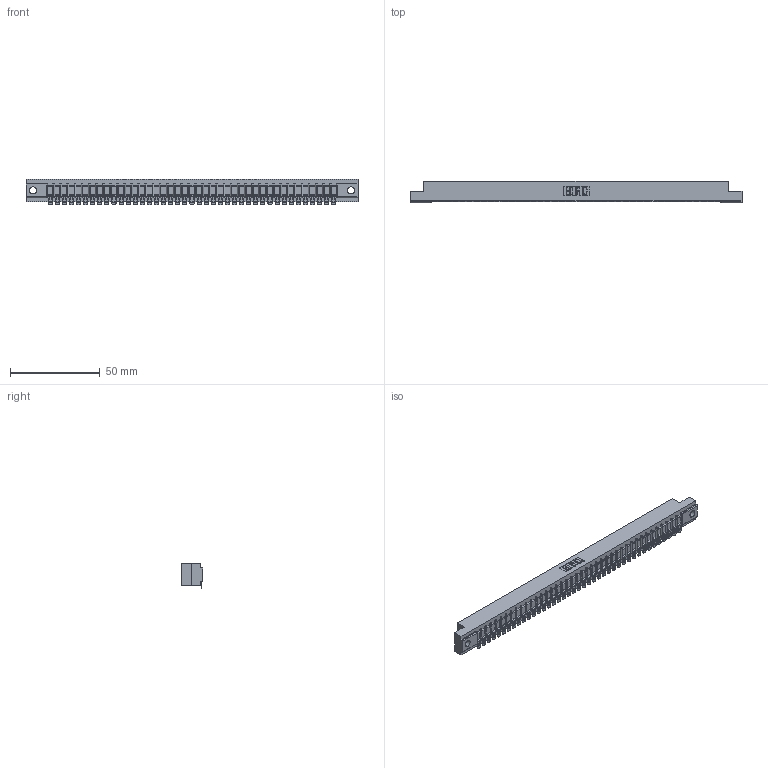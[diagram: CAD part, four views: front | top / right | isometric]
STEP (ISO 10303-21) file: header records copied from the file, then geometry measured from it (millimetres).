
FILE_DESCRIPTION (( 'STEP AP203' ), '1' );
FILE_NAME ('307-041-454-104.STEP', '2020-09-29T16:14:27', ( '' ), ( '' ), 'SwSTEP 2.0', 'SolidWorks 2020', '' );
FILE_SCHEMA (( 'CONFIG_CONTROL_DESIGN' ));
Length unit declared in the file: inch
Products named in the file (3): 307-041-454-104; 307-290-002_554; 307 Part_.156 Dia Mounting Holes
Assembly tree (42 placements, depth 2):
  307-041-454-104
    307 Part_.156 Dia Mounting Holes
    307-290-002_554  x41
Bounding box: 185.47 x 12.01 x 14.52 mm (x, y, z)
Volume: 19749.1 mm3; surface area: 24803.4 mm2
Topology: 42 solids, 42 shells, 3495 faces, 10732 edges, 7040 vertices
Faces by surface type: plane 1970, cylinder 1441, sphere 84
Entity records: 36655 total; most frequent: CARTESIAN_POINT 6188, ORIENTED_EDGE 6176, DIRECTION 6010, EDGE_CURVE 3088, VECTOR 2366, LINE 2366, VERTEX_POINT 2000, AXIS2_PLACEMENT_3D 1822
